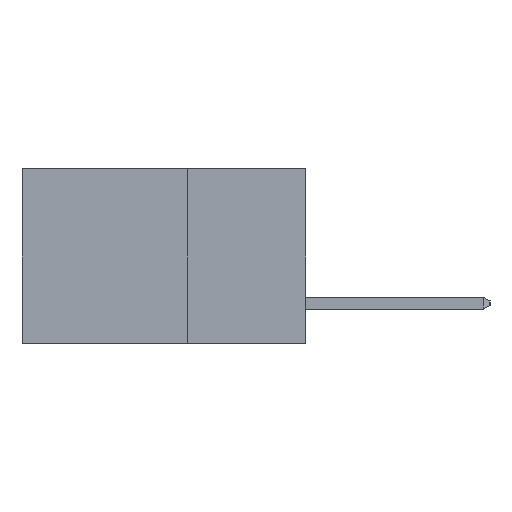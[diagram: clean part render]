
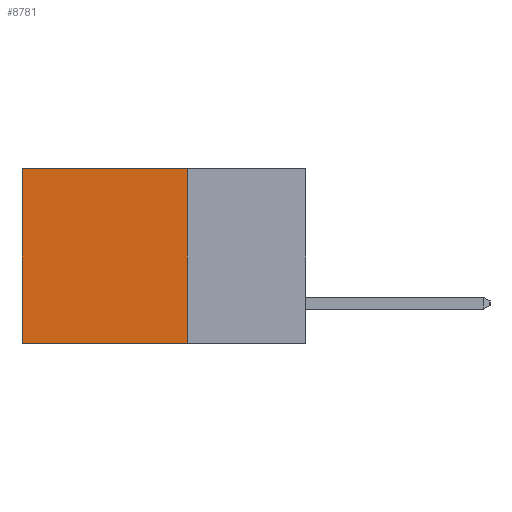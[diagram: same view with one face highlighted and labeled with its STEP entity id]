
A CAD part, left-side view. The second image highlights one B-rep face of the part: STEP entity #8781.
In plain terms, the highlighted planar face has unit normal (-1, 0, 0).
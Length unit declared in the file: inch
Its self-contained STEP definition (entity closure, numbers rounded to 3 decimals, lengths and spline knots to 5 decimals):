
#897 = EDGE_CURVE ( 'NONE', #5693, #8054, #11433, .T. ) ;
#1107 = CARTESIAN_POINT ( 'NONE',  ( 0.2615, 0.25, -0.37 ) ) ;
#1110 = CARTESIAN_POINT ( 'NONE',  ( 0.2615, 0.25, 0. ) ) ;
#1268 = EDGE_CURVE ( 'NONE', #8054, #4473, #2321, .T. ) ;
#1948 = EDGE_LOOP ( 'NONE', ( #10163, #9154, #5072, #7698 ) ) ;
#2040 = AXIS2_PLACEMENT_3D ( 'NONE', #1107, #7611, #2186 ) ;
#2186 = DIRECTION ( 'NONE',  ( 0., 0., -1. ) ) ;
#2321 = LINE ( 'NONE', #6436, #9663 ) ;
#2914 = CARTESIAN_POINT ( 'NONE',  ( 0.2615, 0.6, -0.37 ) ) ;
#3300 = VERTEX_POINT ( 'NONE', #5001 ) ;
#3446 = CARTESIAN_POINT ( 'NONE',  ( 0.2615, 0.25, -0.37 ) ) ;
#3819 = CARTESIAN_POINT ( 'NONE',  ( 0.2615, 0.25, -0.37 ) ) ;
#3928 = CARTESIAN_POINT ( 'NONE',  ( 0.2615, 0.6, 0. ) ) ;
#4376 = DIRECTION ( 'NONE',  ( 0., 0., -1. ) ) ;
#4473 = VERTEX_POINT ( 'NONE', #2914 ) ;
#4859 = LINE ( 'NONE', #3446, #9176 ) ;
#5001 = CARTESIAN_POINT ( 'NONE',  ( 0.2615, 0.25, -0.37 ) ) ;
#5072 = ORIENTED_EDGE ( 'NONE', *, *, #6944, .F. ) ;
#5110 = FACE_OUTER_BOUND ( 'NONE', #1948, .T. ) ;
#5693 = VERTEX_POINT ( 'NONE', #8159 ) ;
#6350 = DIRECTION ( 'NONE',  ( 0., 0., -1. ) ) ;
#6436 = CARTESIAN_POINT ( 'NONE',  ( 0.2615, 0.6, -0.37 ) ) ;
#6482 = EDGE_CURVE ( 'NONE', #3300, #4473, #11107, .T. ) ;
#6614 = VECTOR ( 'NONE', #9839, 39.37008 ) ;
#6721 = PLANE ( 'NONE',  #2040 ) ;
#6944 = EDGE_CURVE ( 'NONE', #5693, #3300, #4859, .T. ) ;
#7300 = DIRECTION ( 'NONE',  ( 0., 1., 0. ) ) ;
#7611 = DIRECTION ( 'NONE',  ( 1., 0., 0. ) ) ;
#7698 = ORIENTED_EDGE ( 'NONE', *, *, #897, .T. ) ;
#8054 = VERTEX_POINT ( 'NONE', #3928 ) ;
#8159 = CARTESIAN_POINT ( 'NONE',  ( 0.2615, 0.25, 0. ) ) ;
#8781 = ADVANCED_FACE ( 'NONE', ( #5110 ), #6721, .F. ) ;
#9154 = ORIENTED_EDGE ( 'NONE', *, *, #6482, .F. ) ;
#9176 = VECTOR ( 'NONE', #4376, 39.37008 ) ;
#9663 = VECTOR ( 'NONE', #6350, 39.37008 ) ;
#9839 = DIRECTION ( 'NONE',  ( 0., 1., 0. ) ) ;
#10163 = ORIENTED_EDGE ( 'NONE', *, *, #1268, .T. ) ;
#11107 = LINE ( 'NONE', #3819, #6614 ) ;
#11217 = VECTOR ( 'NONE', #7300, 39.37008 ) ;
#11433 = LINE ( 'NONE', #1110, #11217 ) ;
